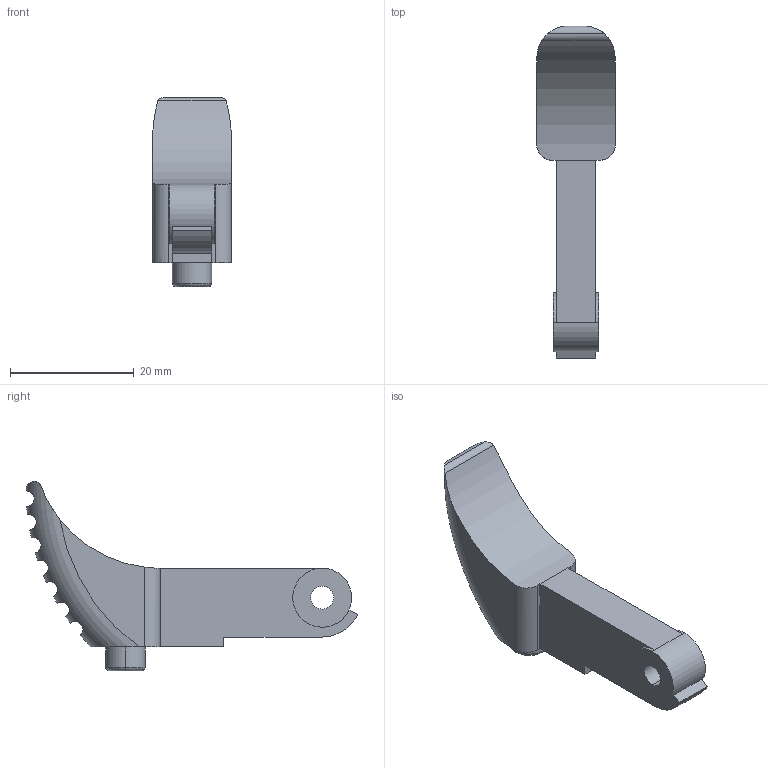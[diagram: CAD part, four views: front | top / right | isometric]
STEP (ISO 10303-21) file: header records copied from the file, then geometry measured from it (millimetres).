
FILE_DESCRIPTION (( 'STEP AP214' ), '1' );
FILE_NAME ('hammer.STEP', '2013-10-27T06:42:32', ( 'Matt' ), ( '' ), 'SwSTEP 2.0', 'SolidWorks 2013', '' );
FILE_SCHEMA (( 'AUTOMOTIVE_DESIGN' ));
Length unit declared in the file: inch
Products named in the file (1): hammer
Bounding box: 12.7 x 53.54 x 30.52 mm (x, y, z)
Volume: 5621.1 mm3; surface area: 2728.5 mm2
Topology: 1 solids, 1 shells, 46 faces, 125 edges, 82 vertices
Faces by surface type: cylinder 28, plane 14, torus 4
Entity records: 1993 total; most frequent: CARTESIAN_POINT 791, ORIENTED_EDGE 250, DIRECTION 240, EDGE_CURVE 125, AXIS2_PLACEMENT_3D 93, VERTEX_POINT 82, LINE 54, VECTOR 54
